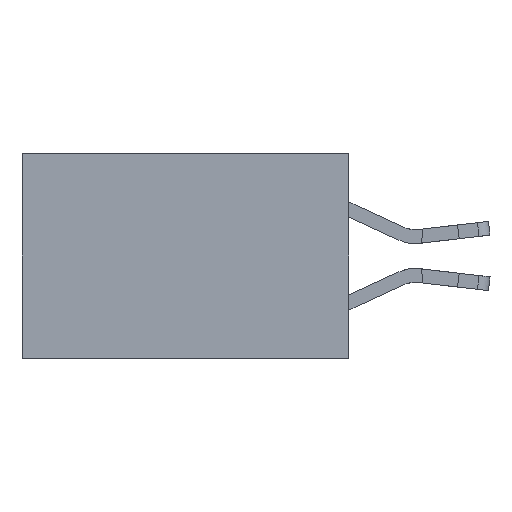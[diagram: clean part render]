
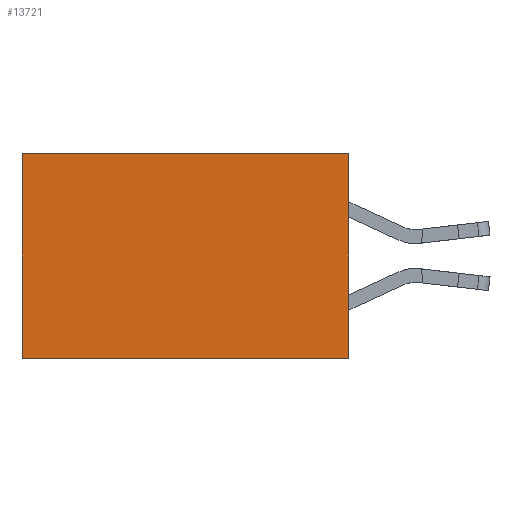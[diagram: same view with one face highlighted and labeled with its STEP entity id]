
A CAD part, left-side view. The second image highlights one B-rep face of the part: STEP entity #13721.
In plain terms, the highlighted planar face has unit normal (-1, 0, 0).
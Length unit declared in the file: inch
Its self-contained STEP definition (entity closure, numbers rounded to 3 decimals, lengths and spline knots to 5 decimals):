
#54 = CARTESIAN_POINT ( 'NONE',  ( 0.277, 0., 0. ) ) ;
#374 = VERTEX_POINT ( 'NONE', #14078 ) ;
#890 = ORIENTED_EDGE ( 'NONE', *, *, #8942, .F. ) ;
#921 = LINE ( 'NONE', #54, #15528 ) ;
#939 = LINE ( 'NONE', #6324, #4243 ) ;
#1146 = DIRECTION ( 'NONE',  ( 1., 0., 0. ) ) ;
#1781 = ORIENTED_EDGE ( 'NONE', *, *, #8162, .T. ) ;
#2622 = EDGE_CURVE ( 'NONE', #4751, #17432, #2750, .T. ) ;
#2625 = VERTEX_POINT ( 'NONE', #13233 ) ;
#2750 = LINE ( 'NONE', #3931, #6558 ) ;
#3931 = CARTESIAN_POINT ( 'NONE',  ( 0.277, 0.59, -0.37 ) ) ;
#4243 = VECTOR ( 'NONE', #14774, 39.37008 ) ;
#4751 = VERTEX_POINT ( 'NONE', #5960 ) ;
#5960 = CARTESIAN_POINT ( 'NONE',  ( 0.277, 0.59, 0. ) ) ;
#6324 = CARTESIAN_POINT ( 'NONE',  ( 0.277, 0., -0.37 ) ) ;
#6558 = VECTOR ( 'NONE', #8859, 39.37008 ) ;
#6936 = LINE ( 'NONE', #17164, #10665 ) ;
#7760 = EDGE_CURVE ( 'NONE', #2625, #17432, #939, .T. ) ;
#8162 = EDGE_CURVE ( 'NONE', #374, #4751, #921, .T. ) ;
#8283 = CARTESIAN_POINT ( 'NONE',  ( 0.277, 0., -0.37 ) ) ;
#8622 = DIRECTION ( 'NONE',  ( 0., 1., 0. ) ) ;
#8845 = DIRECTION ( 'NONE',  ( 0., 0., -1. ) ) ;
#8859 = DIRECTION ( 'NONE',  ( 0., 0., -1. ) ) ;
#8942 = EDGE_CURVE ( 'NONE', #374, #2625, #6936, .T. ) ;
#9671 = PLANE ( 'NONE',  #14683 ) ;
#10613 = FACE_OUTER_BOUND ( 'NONE', #11578, .T. ) ;
#10665 = VECTOR ( 'NONE', #8845, 39.37008 ) ;
#11081 = DIRECTION ( 'NONE',  ( 0., 0., -1. ) ) ;
#11578 = EDGE_LOOP ( 'NONE', ( #13476, #12945, #890, #1781 ) ) ;
#12945 = ORIENTED_EDGE ( 'NONE', *, *, #7760, .F. ) ;
#13233 = CARTESIAN_POINT ( 'NONE',  ( 0.277, 0., -0.37 ) ) ;
#13476 = ORIENTED_EDGE ( 'NONE', *, *, #2622, .T. ) ;
#13721 = ADVANCED_FACE ( 'NONE', ( #10613 ), #9671, .F. ) ;
#14078 = CARTESIAN_POINT ( 'NONE',  ( 0.277, 0., 0. ) ) ;
#14683 = AXIS2_PLACEMENT_3D ( 'NONE', #8283, #1146, #11081 ) ;
#14774 = DIRECTION ( 'NONE',  ( 0., 1., 0. ) ) ;
#15528 = VECTOR ( 'NONE', #8622, 39.37008 ) ;
#16137 = CARTESIAN_POINT ( 'NONE',  ( 0.277, 0.59, -0.37 ) ) ;
#17164 = CARTESIAN_POINT ( 'NONE',  ( 0.277, 0., -0.37 ) ) ;
#17432 = VERTEX_POINT ( 'NONE', #16137 ) ;
